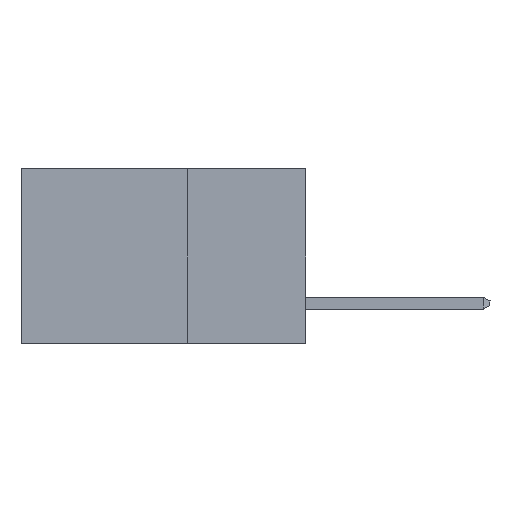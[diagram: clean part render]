
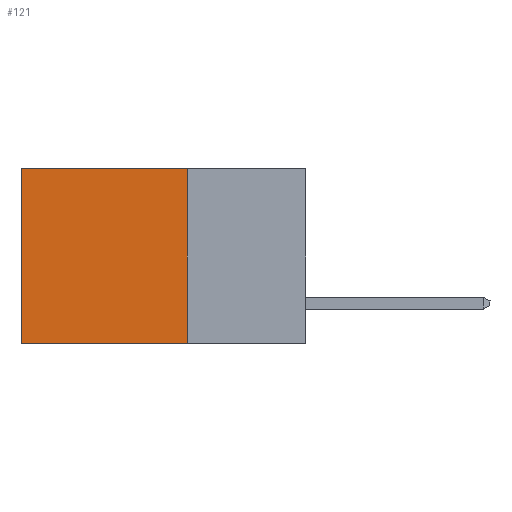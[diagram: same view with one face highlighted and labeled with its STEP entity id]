
A CAD part, left-side view. The second image highlights one B-rep face of the part: STEP entity #121.
In plain terms, the highlighted planar face has unit normal (-1, 0, 0).
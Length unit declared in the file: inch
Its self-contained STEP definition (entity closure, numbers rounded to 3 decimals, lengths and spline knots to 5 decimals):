
#121 = ADVANCED_FACE ( 'NONE', ( #3310 ), #6784, .F. ) ;
#969 = LINE ( 'NONE', #7898, #6166 ) ;
#998 = ORIENTED_EDGE ( 'NONE', *, *, #1895, .T. ) ;
#1097 = ORIENTED_EDGE ( 'NONE', *, *, #10084, .F. ) ;
#1149 = LINE ( 'NONE', #2744, #7299 ) ;
#1537 = VERTEX_POINT ( 'NONE', #9185 ) ;
#1895 = EDGE_CURVE ( 'NONE', #6998, #3172, #9971, .T. ) ;
#2730 = DIRECTION ( 'NONE',  ( 0., 1., 0. ) ) ;
#2744 = CARTESIAN_POINT ( 'NONE',  ( 0.2615, 0.25, -0.37 ) ) ;
#3172 = VERTEX_POINT ( 'NONE', #6444 ) ;
#3203 = VECTOR ( 'NONE', #7351, 39.37008 ) ;
#3310 = FACE_OUTER_BOUND ( 'NONE', #9944, .T. ) ;
#3424 = DIRECTION ( 'NONE',  ( 0., 0., -1. ) ) ;
#4586 = EDGE_CURVE ( 'NONE', #1537, #6998, #969, .T. ) ;
#4681 = DIRECTION ( 'NONE',  ( 0., 1., 0. ) ) ;
#5020 = CARTESIAN_POINT ( 'NONE',  ( 0.2615, 0.25, -0.37 ) ) ;
#5066 = CARTESIAN_POINT ( 'NONE',  ( 0.2615, 0.6, 0. ) ) ;
#5319 = VERTEX_POINT ( 'NONE', #5020 ) ;
#5366 = LINE ( 'NONE', #8045, #8943 ) ;
#5490 = DIRECTION ( 'NONE',  ( 0., 0., -1. ) ) ;
#6166 = VECTOR ( 'NONE', #2730, 39.37008 ) ;
#6423 = ORIENTED_EDGE ( 'NONE', *, *, #9526, .F. ) ;
#6444 = CARTESIAN_POINT ( 'NONE',  ( 0.2615, 0.6, -0.37 ) ) ;
#6784 = PLANE ( 'NONE',  #7017 ) ;
#6998 = VERTEX_POINT ( 'NONE', #5066 ) ;
#7017 = AXIS2_PLACEMENT_3D ( 'NONE', #10257, #11228, #3424 ) ;
#7299 = VECTOR ( 'NONE', #4681, 39.37008 ) ;
#7351 = DIRECTION ( 'NONE',  ( 0., 0., -1. ) ) ;
#7898 = CARTESIAN_POINT ( 'NONE',  ( 0.2615, 0.25, 0. ) ) ;
#8045 = CARTESIAN_POINT ( 'NONE',  ( 0.2615, 0.25, -0.37 ) ) ;
#8943 = VECTOR ( 'NONE', #5490, 39.37008 ) ;
#9185 = CARTESIAN_POINT ( 'NONE',  ( 0.2615, 0.25, 0. ) ) ;
#9526 = EDGE_CURVE ( 'NONE', #1537, #5319, #5366, .T. ) ;
#9944 = EDGE_LOOP ( 'NONE', ( #998, #1097, #6423, #10425 ) ) ;
#9971 = LINE ( 'NONE', #10078, #3203 ) ;
#10078 = CARTESIAN_POINT ( 'NONE',  ( 0.2615, 0.6, -0.37 ) ) ;
#10084 = EDGE_CURVE ( 'NONE', #5319, #3172, #1149, .T. ) ;
#10257 = CARTESIAN_POINT ( 'NONE',  ( 0.2615, 0.25, -0.37 ) ) ;
#10425 = ORIENTED_EDGE ( 'NONE', *, *, #4586, .T. ) ;
#11228 = DIRECTION ( 'NONE',  ( 1., 0., 0. ) ) ;
